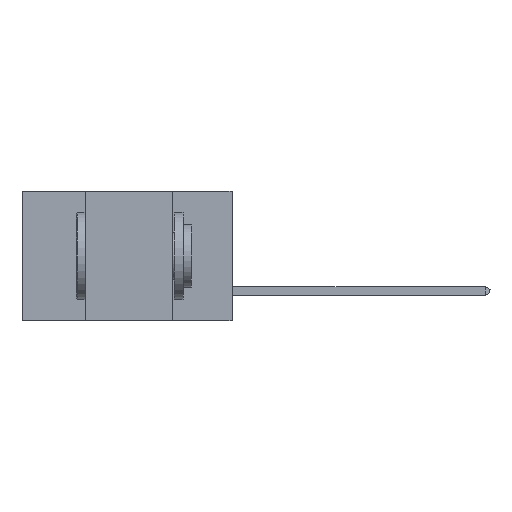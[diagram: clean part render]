
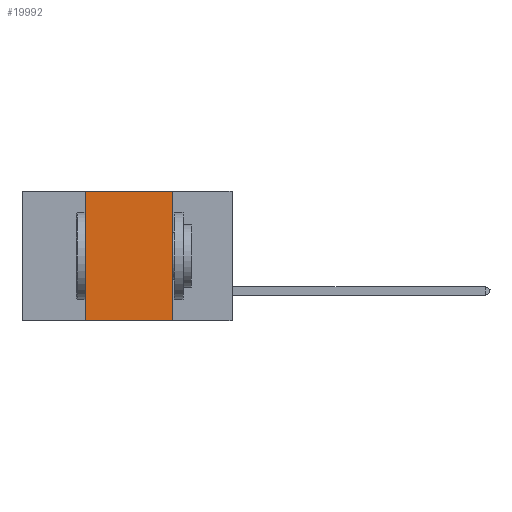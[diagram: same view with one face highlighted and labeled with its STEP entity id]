
A CAD part, left-side view. The second image highlights one B-rep face of the part: STEP entity #19992.
In plain terms, the highlighted planar face has unit normal (-1, 0, 0).
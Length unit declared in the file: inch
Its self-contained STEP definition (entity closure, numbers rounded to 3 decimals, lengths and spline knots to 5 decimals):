
#2555 = DIRECTION ( 'NONE',  ( 0., 0., 1. ) ) ;
#3450 = VECTOR ( 'NONE', #19602, 39.37008 ) ;
#4230 = CARTESIAN_POINT ( 'NONE',  ( 0., 0.17, 0. ) ) ;
#4728 = VERTEX_POINT ( 'NONE', #20537 ) ;
#5740 = CARTESIAN_POINT ( 'NONE',  ( 0., 0.17, 0. ) ) ;
#6104 = EDGE_CURVE ( 'NONE', #9244, #13453, #8824, .T. ) ;
#6208 = CARTESIAN_POINT ( 'NONE',  ( 0., 0.6, -0.37 ) ) ;
#6723 = LINE ( 'NONE', #6208, #10121 ) ;
#6756 = EDGE_CURVE ( 'NONE', #13453, #4728, #24120, .T. ) ;
#8459 = EDGE_CURVE ( 'NONE', #17424, #9244, #19301, .T. ) ;
#8824 = LINE ( 'NONE', #9787, #3450 ) ;
#9001 = DIRECTION ( 'NONE',  ( 0., 0., -1. ) ) ;
#9024 = CARTESIAN_POINT ( 'NONE',  ( 0., 0.42, -0.37 ) ) ;
#9244 = VERTEX_POINT ( 'NONE', #21398 ) ;
#9787 = CARTESIAN_POINT ( 'NONE',  ( 0., 0.6, 0. ) ) ;
#10121 = VECTOR ( 'NONE', #10352, 39.37008 ) ;
#10352 = DIRECTION ( 'NONE',  ( 0., -1., 0. ) ) ;
#11124 = DIRECTION ( 'NONE',  ( 1., 0., 0. ) ) ;
#11159 = AXIS2_PLACEMENT_3D ( 'NONE', #19203, #11124, #9001 ) ;
#11922 = ORIENTED_EDGE ( 'NONE', *, *, #17386, .T. ) ;
#13453 = VERTEX_POINT ( 'NONE', #4230 ) ;
#15169 = EDGE_LOOP ( 'NONE', ( #19972, #24075, #24714, #11922 ) ) ;
#17386 = EDGE_CURVE ( 'NONE', #17424, #4728, #6723, .T. ) ;
#17424 = VERTEX_POINT ( 'NONE', #9024 ) ;
#18661 = VECTOR ( 'NONE', #2555, 39.37008 ) ;
#19203 = CARTESIAN_POINT ( 'NONE',  ( 0., 0.6, 0. ) ) ;
#19301 = LINE ( 'NONE', #24709, #18661 ) ;
#19602 = DIRECTION ( 'NONE',  ( 0., -1., 0. ) ) ;
#19972 = ORIENTED_EDGE ( 'NONE', *, *, #6756, .F. ) ;
#19992 = ADVANCED_FACE ( 'NONE', ( #25057 ), #25120, .F. ) ;
#20537 = CARTESIAN_POINT ( 'NONE',  ( 0., 0.17, -0.37 ) ) ;
#21398 = CARTESIAN_POINT ( 'NONE',  ( 0., 0.42, 0. ) ) ;
#22547 = VECTOR ( 'NONE', #23951, 39.37008 ) ;
#23951 = DIRECTION ( 'NONE',  ( 0., 0., -1. ) ) ;
#24075 = ORIENTED_EDGE ( 'NONE', *, *, #6104, .F. ) ;
#24120 = LINE ( 'NONE', #5740, #22547 ) ;
#24709 = CARTESIAN_POINT ( 'NONE',  ( 0., 0.42, 0. ) ) ;
#24714 = ORIENTED_EDGE ( 'NONE', *, *, #8459, .F. ) ;
#25057 = FACE_OUTER_BOUND ( 'NONE', #15169, .T. ) ;
#25120 = PLANE ( 'NONE',  #11159 ) ;
